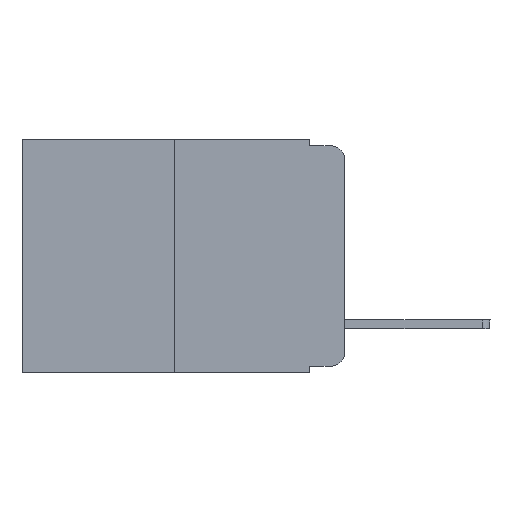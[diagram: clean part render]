
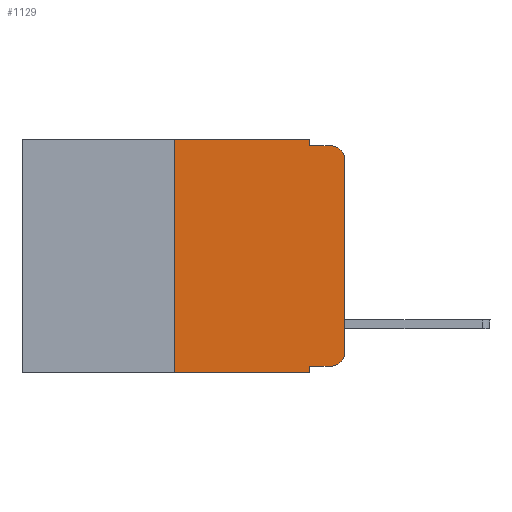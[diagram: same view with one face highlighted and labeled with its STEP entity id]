
A CAD part, left-side view. The second image highlights one B-rep face of the part: STEP entity #1129.
In plain terms, the highlighted planar face has unit normal (-1, 0, 0).
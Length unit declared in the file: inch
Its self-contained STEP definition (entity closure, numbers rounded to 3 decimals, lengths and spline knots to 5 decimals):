
#36 = ORIENTED_EDGE ( 'NONE', *, *, #3026, .F. ) ;
#198 = CIRCLE ( 'NONE', #3695, 0.02 ) ;
#212 = CARTESIAN_POINT ( 'NONE',  ( 0., 0., -0.313 ) ) ;
#235 = LINE ( 'NONE', #1057, #3328 ) ;
#269 = DIRECTION ( 'NONE',  ( 0., 0., 1. ) ) ;
#322 = ORIENTED_EDGE ( 'NONE', *, *, #1720, .F. ) ;
#473 = VERTEX_POINT ( 'NONE', #7508 ) ;
#599 = DIRECTION ( 'NONE',  ( 0., 0., -1. ) ) ;
#636 = DIRECTION ( 'NONE',  ( 0., -1., 0. ) ) ;
#901 = DIRECTION ( 'NONE',  ( 0., 0., -1. ) ) ;
#1057 = CARTESIAN_POINT ( 'NONE',  ( 0., 0.051, 0. ) ) ;
#1088 = AXIS2_PLACEMENT_3D ( 'NONE', #7989, #6442, #901 ) ;
#1124 = LINE ( 'NONE', #8157, #7361 ) ;
#1129 = ADVANCED_FACE ( 'NONE', ( #4814 ), #6584, .F. ) ;
#1301 = VERTEX_POINT ( 'NONE', #8304 ) ;
#1363 = LINE ( 'NONE', #3131, #5433 ) ;
#1447 = EDGE_CURVE ( 'NONE', #1301, #1525, #1363, .T. ) ;
#1453 = DIRECTION ( 'NONE',  ( 0., -1., 0. ) ) ;
#1467 = DIRECTION ( 'NONE',  ( 0., -1., 0. ) ) ;
#1524 = VERTEX_POINT ( 'NONE', #212 ) ;
#1525 = VERTEX_POINT ( 'NONE', #9637 ) ;
#1570 = LINE ( 'NONE', #4558, #2133 ) ;
#1720 = EDGE_CURVE ( 'NONE', #2027, #8922, #2041, .T. ) ;
#1866 = ORIENTED_EDGE ( 'NONE', *, *, #2028, .T. ) ;
#1921 = CIRCLE ( 'NONE', #7254, 0.02 ) ;
#1943 = DIRECTION ( 'NONE',  ( -1., 0., 0. ) ) ;
#2027 = VERTEX_POINT ( 'NONE', #3267 ) ;
#2028 = EDGE_CURVE ( 'NONE', #473, #8278, #8070, .T. ) ;
#2041 = LINE ( 'NONE', #4440, #9750 ) ;
#2133 = VECTOR ( 'NONE', #1467, 39.37008 ) ;
#2278 = ORIENTED_EDGE ( 'NONE', *, *, #5486, .F. ) ;
#2677 = CARTESIAN_POINT ( 'NONE',  ( 0., 0.051, -0.343 ) ) ;
#3019 = CARTESIAN_POINT ( 'NONE',  ( 0., 0.02, -0.01 ) ) ;
#3026 = EDGE_CURVE ( 'NONE', #8922, #1301, #9279, .T. ) ;
#3107 = VECTOR ( 'NONE', #5670, 39.37008 ) ;
#3131 = CARTESIAN_POINT ( 'NONE',  ( 0., 0.051, 0. ) ) ;
#3267 = CARTESIAN_POINT ( 'NONE',  ( 0., 0.25, -0.343 ) ) ;
#3328 = VECTOR ( 'NONE', #3402, 39.37008 ) ;
#3402 = DIRECTION ( 'NONE',  ( 0., 0., -1. ) ) ;
#3680 = DIRECTION ( 'NONE',  ( -1., 0., 0. ) ) ;
#3695 = AXIS2_PLACEMENT_3D ( 'NONE', #6689, #1943, #8296 ) ;
#4135 = ORIENTED_EDGE ( 'NONE', *, *, #8846, .T. ) ;
#4440 = CARTESIAN_POINT ( 'NONE',  ( 0., 0.25, 0. ) ) ;
#4558 = CARTESIAN_POINT ( 'NONE',  ( 0., 0.051, -0.01 ) ) ;
#4737 = LINE ( 'NONE', #8596, #8048 ) ;
#4814 = FACE_OUTER_BOUND ( 'NONE', #9496, .T. ) ;
#4901 = CARTESIAN_POINT ( 'NONE',  ( 0., 0.02, -0.333 ) ) ;
#4909 = VERTEX_POINT ( 'NONE', #2677 ) ;
#5317 = CARTESIAN_POINT ( 'NONE',  ( 0., 0.473, 0. ) ) ;
#5433 = VECTOR ( 'NONE', #599, 39.37008 ) ;
#5486 = EDGE_CURVE ( 'NONE', #1525, #5498, #1570, .T. ) ;
#5498 = VERTEX_POINT ( 'NONE', #3019 ) ;
#5670 = DIRECTION ( 'NONE',  ( 0., -1., 0. ) ) ;
#6315 = EDGE_CURVE ( 'NONE', #8278, #1524, #1921, .T. ) ;
#6442 = DIRECTION ( 'NONE',  ( 1., 0., 0. ) ) ;
#6584 = PLANE ( 'NONE',  #1088 ) ;
#6597 = ORIENTED_EDGE ( 'NONE', *, *, #6620, .F. ) ;
#6603 = DIRECTION ( 'NONE',  ( 0., 0., 1. ) ) ;
#6620 = EDGE_CURVE ( 'NONE', #473, #4909, #235, .T. ) ;
#6683 = VERTEX_POINT ( 'NONE', #7737 ) ;
#6689 = CARTESIAN_POINT ( 'NONE',  ( 0., 0.02, -0.03 ) ) ;
#7033 = CARTESIAN_POINT ( 'NONE',  ( 0., 0.02, -0.313 ) ) ;
#7194 = CARTESIAN_POINT ( 'NONE',  ( 0., 0.051, -0.333 ) ) ;
#7254 = AXIS2_PLACEMENT_3D ( 'NONE', #7033, #3680, #10206 ) ;
#7361 = VECTOR ( 'NONE', #6603, 39.37008 ) ;
#7508 = CARTESIAN_POINT ( 'NONE',  ( 0., 0.051, -0.333 ) ) ;
#7737 = CARTESIAN_POINT ( 'NONE',  ( 0., 0., -0.03 ) ) ;
#7806 = VECTOR ( 'NONE', #636, 39.37008 ) ;
#7976 = ORIENTED_EDGE ( 'NONE', *, *, #8185, .T. ) ;
#7989 = CARTESIAN_POINT ( 'NONE',  ( 0., 0.473, 0. ) ) ;
#8048 = VECTOR ( 'NONE', #1453, 39.37008 ) ;
#8070 = LINE ( 'NONE', #7194, #3107 ) ;
#8157 = CARTESIAN_POINT ( 'NONE',  ( 0., 0., 0. ) ) ;
#8185 = EDGE_CURVE ( 'NONE', #6683, #5498, #198, .T. ) ;
#8278 = VERTEX_POINT ( 'NONE', #4901 ) ;
#8296 = DIRECTION ( 'NONE',  ( 0., 0., -1. ) ) ;
#8304 = CARTESIAN_POINT ( 'NONE',  ( 0., 0.051, 0. ) ) ;
#8391 = ORIENTED_EDGE ( 'NONE', *, *, #9734, .T. ) ;
#8596 = CARTESIAN_POINT ( 'NONE',  ( 0., 0.473, -0.343 ) ) ;
#8846 = EDGE_CURVE ( 'NONE', #1524, #6683, #1124, .T. ) ;
#8922 = VERTEX_POINT ( 'NONE', #9204 ) ;
#9204 = CARTESIAN_POINT ( 'NONE',  ( 0., 0.25, 0. ) ) ;
#9279 = LINE ( 'NONE', #5317, #7806 ) ;
#9496 = EDGE_LOOP ( 'NONE', ( #4135, #7976, #2278, #9694, #36, #322, #8391, #6597, #1866, #9857 ) ) ;
#9637 = CARTESIAN_POINT ( 'NONE',  ( 0., 0.051, -0.01 ) ) ;
#9694 = ORIENTED_EDGE ( 'NONE', *, *, #1447, .F. ) ;
#9734 = EDGE_CURVE ( 'NONE', #2027, #4909, #4737, .T. ) ;
#9750 = VECTOR ( 'NONE', #269, 39.37008 ) ;
#9857 = ORIENTED_EDGE ( 'NONE', *, *, #6315, .T. ) ;
#10206 = DIRECTION ( 'NONE',  ( 0., 0., -1. ) ) ;
